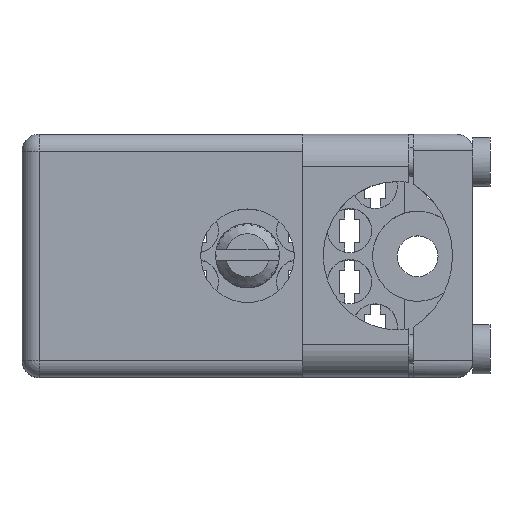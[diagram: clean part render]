
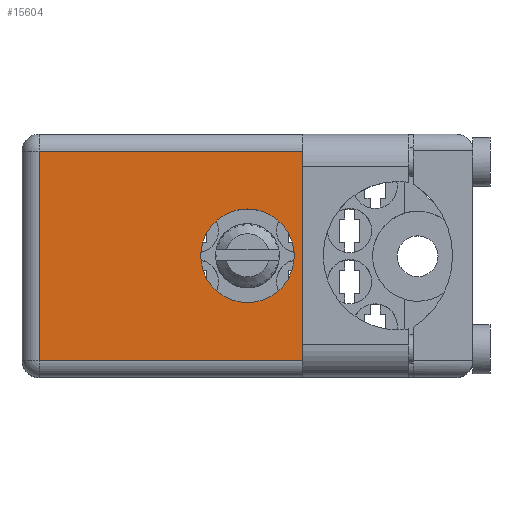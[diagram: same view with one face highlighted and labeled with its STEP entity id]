
A CAD part, top view. The second image highlights one B-rep face of the part: STEP entity #15604.
In plain terms, the highlighted face is planar.
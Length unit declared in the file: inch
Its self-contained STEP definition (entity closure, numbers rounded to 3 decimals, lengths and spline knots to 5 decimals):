
#5810 = DIRECTION ( 'NONE',  ( 0., 0., -1. ) ) ;
#8230 = EDGE_CURVE ( 'NONE', #130954, #41860, #144522, .T. ) ;
#8940 = CARTESIAN_POINT ( 'NONE',  ( 1.15, 0.906, -0.6025 ) ) ;
#9364 = VECTOR ( 'NONE', #137763, 39.37008 ) ;
#12693 = VERTEX_POINT ( 'NONE', #88888 ) ;
#13453 = CARTESIAN_POINT ( 'NONE',  ( 0., 0.906, -0.715 ) ) ;
#15604 = ADVANCED_FACE ( 'NONE', ( #75958, #105246 ), #157022, .T. ) ;
#21520 = EDGE_CURVE ( 'NONE', #149795, #130954, #87825, .T. ) ;
#23136 = DIRECTION ( 'NONE',  ( 0., 1., 0. ) ) ;
#25867 = LINE ( 'NONE', #85399, #136177 ) ;
#26030 = VERTEX_POINT ( 'NONE', #8940 ) ;
#26361 = VECTOR ( 'NONE', #127060, 39.37008 ) ;
#26915 = DIRECTION ( 'NONE',  ( -1., 0., 0. ) ) ;
#27063 = CARTESIAN_POINT ( 'NONE',  ( 1.15, 0.906, -0.715 ) ) ;
#31477 = VERTEX_POINT ( 'NONE', #69259 ) ;
#32342 = ORIENTED_EDGE ( 'NONE', *, *, #21520, .T. ) ;
#33448 = ORIENTED_EDGE ( 'NONE', *, *, #139554, .T. ) ;
#36744 = CARTESIAN_POINT ( 'NONE',  ( 0.865, 0.906, -0.1125 ) ) ;
#37746 = CARTESIAN_POINT ( 'NONE',  ( 1.15, 0.906, -0.715 ) ) ;
#38905 = VERTEX_POINT ( 'NONE', #159515 ) ;
#39635 = DIRECTION ( 'NONE',  ( -1., 0., 0. ) ) ;
#40634 = VECTOR ( 'NONE', #39635, 39.37008 ) ;
#41860 = VERTEX_POINT ( 'NONE', #168739 ) ;
#45288 = EDGE_LOOP ( 'NONE', ( #50176, #184083 ) ) ;
#49612 = CARTESIAN_POINT ( 'NONE',  ( 0.6625, 0.906, -0.3575 ) ) ;
#50176 = ORIENTED_EDGE ( 'NONE', *, *, #98847, .F. ) ;
#64920 = DIRECTION ( 'NONE',  ( 0., 0., 1. ) ) ;
#67681 = LINE ( 'NONE', #95011, #40634 ) ;
#69259 = CARTESIAN_POINT ( 'NONE',  ( 0.865, 0.906, -0.6025 ) ) ;
#69752 = CARTESIAN_POINT ( 'NONE',  ( 0.865, 0.906, -0.1125 ) ) ;
#70329 = ORIENTED_EDGE ( 'NONE', *, *, #98283, .F. ) ;
#75200 = ORIENTED_EDGE ( 'NONE', *, *, #179838, .F. ) ;
#75613 = CARTESIAN_POINT ( 'NONE',  ( 0.6625, 0.906, -0.22 ) ) ;
#75958 = FACE_OUTER_BOUND ( 'NONE', #95180, .T. ) ;
#78113 = AXIS2_PLACEMENT_3D ( 'NONE', #153015, #136659, #64920 ) ;
#78996 = DIRECTION ( 'NONE',  ( 1., 0., 0. ) ) ;
#81838 = LINE ( 'NONE', #121768, #88481 ) ;
#85399 = CARTESIAN_POINT ( 'NONE',  ( 0.865, 0.906, -0.1125 ) ) ;
#85861 = DIRECTION ( 'NONE',  ( 0., 1., 0. ) ) ;
#87825 = LINE ( 'NONE', #181679, #150893 ) ;
#88481 = VECTOR ( 'NONE', #78996, 39.37008 ) ;
#88888 = CARTESIAN_POINT ( 'NONE',  ( 1.15, 0.906, -0.665 ) ) ;
#89538 = VERTEX_POINT ( 'NONE', #75613 ) ;
#91677 = ORIENTED_EDGE ( 'NONE', *, *, #112642, .T. ) ;
#92123 = AXIS2_PLACEMENT_3D ( 'NONE', #13453, #85861, #114223 ) ;
#92986 = DIRECTION ( 'NONE',  ( 0., 0., 1. ) ) ;
#95011 = CARTESIAN_POINT ( 'NONE',  ( 0., 0.906, -0.665 ) ) ;
#95180 = EDGE_LOOP ( 'NONE', ( #32342, #153002, #75200, #33448, #91677, #106572, #70329, #98054 ) ) ;
#95331 = AXIS2_PLACEMENT_3D ( 'NONE', #49612, #23136, #92986 ) ;
#95403 = DIRECTION ( 'NONE',  ( 0., 0., 1. ) ) ;
#96203 = CARTESIAN_POINT ( 'NONE',  ( 1.15, 0.906, -0.05 ) ) ;
#98054 = ORIENTED_EDGE ( 'NONE', *, *, #149276, .T. ) ;
#98283 = EDGE_CURVE ( 'NONE', #12693, #26030, #162756, .T. ) ;
#98847 = EDGE_CURVE ( 'NONE', #89538, #104028, #153776, .T. ) ;
#104028 = VERTEX_POINT ( 'NONE', #105866 ) ;
#105246 = FACE_BOUND ( 'NONE', #45288, .T. ) ;
#105866 = CARTESIAN_POINT ( 'NONE',  ( 0.6625, 0.906, -0.495 ) ) ;
#106110 = VERTEX_POINT ( 'NONE', #69752 ) ;
#106572 = ORIENTED_EDGE ( 'NONE', *, *, #160406, .T. ) ;
#112642 = EDGE_CURVE ( 'NONE', #106110, #31477, #120204, .T. ) ;
#114223 = DIRECTION ( 'NONE',  ( 0., 0., 1. ) ) ;
#120204 = LINE ( 'NONE', #36744, #149520 ) ;
#121768 = CARTESIAN_POINT ( 'NONE',  ( 0.865, 0.906, -0.6025 ) ) ;
#127060 = DIRECTION ( 'NONE',  ( 0., 0., 1. ) ) ;
#130954 = VERTEX_POINT ( 'NONE', #175791 ) ;
#136177 = VECTOR ( 'NONE', #26915, 39.37008 ) ;
#136659 = DIRECTION ( 'NONE',  ( 0., 1., 0. ) ) ;
#137763 = DIRECTION ( 'NONE',  ( 1., 0., 0. ) ) ;
#139494 = CARTESIAN_POINT ( 'NONE',  ( 0.05, 0.906, -0.665 ) ) ;
#139554 = EDGE_CURVE ( 'NONE', #38905, #106110, #25867, .T. ) ;
#144522 = LINE ( 'NONE', #96203, #9364 ) ;
#149276 = EDGE_CURVE ( 'NONE', #12693, #149795, #67681, .T. ) ;
#149520 = VECTOR ( 'NONE', #5810, 39.37008 ) ;
#149795 = VERTEX_POINT ( 'NONE', #139494 ) ;
#150893 = VECTOR ( 'NONE', #95403, 39.37008 ) ;
#153002 = ORIENTED_EDGE ( 'NONE', *, *, #8230, .T. ) ;
#153015 = CARTESIAN_POINT ( 'NONE',  ( 0.6625, 0.906, -0.3575 ) ) ;
#153776 = CIRCLE ( 'NONE', #95331, 0.1375 ) ;
#157022 = PLANE ( 'NONE',  #92123 ) ;
#159515 = CARTESIAN_POINT ( 'NONE',  ( 1.15, 0.906, -0.1125 ) ) ;
#160406 = EDGE_CURVE ( 'NONE', #31477, #26030, #81838, .T. ) ;
#160496 = CIRCLE ( 'NONE', #78113, 0.1375 ) ;
#162756 = LINE ( 'NONE', #37746, #180916 ) ;
#167952 = DIRECTION ( 'NONE',  ( 0., 0., 1. ) ) ;
#168739 = CARTESIAN_POINT ( 'NONE',  ( 1.15, 0.906, -0.05 ) ) ;
#170226 = LINE ( 'NONE', #27063, #26361 ) ;
#175791 = CARTESIAN_POINT ( 'NONE',  ( 0.05, 0.906, -0.05 ) ) ;
#176138 = EDGE_CURVE ( 'NONE', #104028, #89538, #160496, .T. ) ;
#179838 = EDGE_CURVE ( 'NONE', #38905, #41860, #170226, .T. ) ;
#180916 = VECTOR ( 'NONE', #167952, 39.37008 ) ;
#181679 = CARTESIAN_POINT ( 'NONE',  ( 0.05, 0.906, -0.715 ) ) ;
#184083 = ORIENTED_EDGE ( 'NONE', *, *, #176138, .F. ) ;
